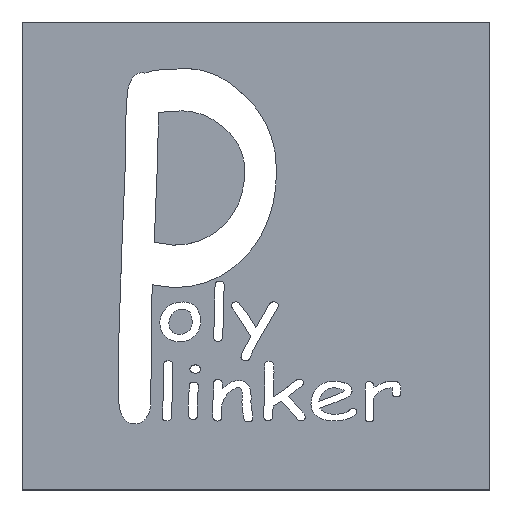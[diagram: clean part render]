
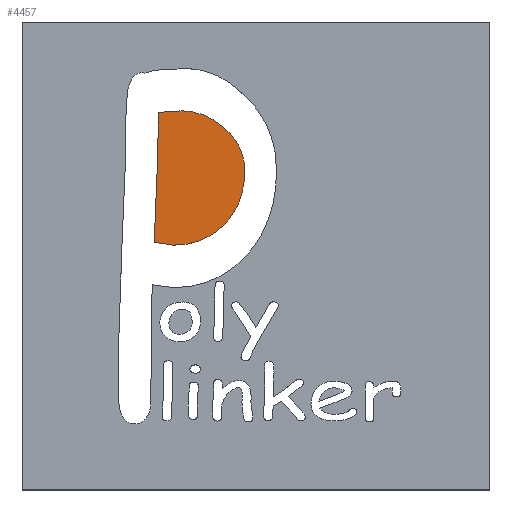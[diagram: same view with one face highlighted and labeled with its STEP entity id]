
A CAD part, top view. The second image highlights one B-rep face of the part: STEP entity #4457.
In plain terms, the highlighted planar face has unit normal (0, 0, 1).
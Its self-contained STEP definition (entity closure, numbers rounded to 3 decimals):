
#68 = EDGE_CURVE ( 'NONE', #655, #737, #5095, .T. ) ;
#99 = FACE_OUTER_BOUND ( 'NONE', #6360, .T. ) ;
#329 = B_SPLINE_CURVE_WITH_KNOTS ( 'NONE', 3,
 ( #1720, #4419, #2565, #1857 ),
 .UNSPECIFIED., .F., .F.,
 ( 4, 4 ),
 ( 0., 1. ),
 .UNSPECIFIED. ) ;
#407 = CARTESIAN_POINT ( 'NONE',  ( -11.199, 9.246, 22.127 ) ) ;
#552 = VECTOR ( 'NONE', #1691, 1000. ) ;
#575 = VECTOR ( 'NONE', #4818, 1000. ) ;
#655 = VERTEX_POINT ( 'NONE', #2930 ) ;
#659 = CARTESIAN_POINT ( 'NONE',  ( -5.569, 11.492, 22.127 ) ) ;
#734 = CARTESIAN_POINT ( 'NONE',  ( -10.305, 12.862, 22.127 ) ) ;
#737 = VERTEX_POINT ( 'NONE', #407 ) ;
#823 = EDGE_CURVE ( 'NONE', #4748, #655, #2637, .T. ) ;
#871 = EDGE_CURVE ( 'NONE', #737, #2828, #1374, .T. ) ;
#1062 = CARTESIAN_POINT ( 'NONE',  ( -7.858, 12.9, 22.127 ) ) ;
#1065 = ORIENTED_EDGE ( 'NONE', *, *, #4635, .T. ) ;
#1147 = EDGE_CURVE ( 'NONE', #3912, #3196, #5154, .T. ) ;
#1374 = LINE ( 'NONE', #3438, #575 ) ;
#1389 = DIRECTION ( 'NONE',  ( 0., 0., -1. ) ) ;
#1469 = DIRECTION ( 'NONE',  ( -1., 0., 0. ) ) ;
#1534 = CARTESIAN_POINT ( 'NONE',  ( -11.511, 1.673, 22.127 ) ) ;
#1585 = EDGE_CURVE ( 'NONE', #2828, #3912, #5687, .T. ) ;
#1691 = DIRECTION ( 'NONE',  ( -0.009, -1., 0. ) ) ;
#1720 = CARTESIAN_POINT ( 'NONE',  ( -5.658, 3.043, 22.127 ) ) ;
#1794 = CARTESIAN_POINT ( 'NONE',  ( -5.658, 3.043, 22.127 ) ) ;
#1857 = CARTESIAN_POINT ( 'NONE',  ( -3.782, 7.819, 22.127 ) ) ;
#1935 = CARTESIAN_POINT ( 'NONE',  ( -5.569, 11.492, 22.127 ) ) ;
#2131 = CARTESIAN_POINT ( 'NONE',  ( 0., 22.127, 22.127 ) ) ;
#2137 = B_SPLINE_CURVE_WITH_KNOTS ( 'NONE', 3,
 ( #8419, #7103, #1062, #7329 ),
 .UNSPECIFIED., .F., .F.,
 ( 4, 4 ),
 ( 0., 1. ),
 .UNSPECIFIED. ) ;
#2221 = CARTESIAN_POINT ( 'NONE',  ( -9.565, 12.9, 22.127 ) ) ;
#2227 = ORIENTED_EDGE ( 'NONE', *, *, #5098, .T. ) ;
#2451 = CARTESIAN_POINT ( 'NONE',  ( -6.8, 1.965, 22.127 ) ) ;
#2565 = CARTESIAN_POINT ( 'NONE',  ( -3.782, 5.815, 22.127 ) ) ;
#2591 = CARTESIAN_POINT ( 'NONE',  ( -8.205, 1.425, 22.127 ) ) ;
#2606 = CARTESIAN_POINT ( 'NONE',  ( -11.511, 1.673, 22.127 ) ) ;
#2637 = B_SPLINE_CURVE_WITH_KNOTS ( 'NONE', 3,
 ( #5141, #7816, #6682, #4480 ),
 .UNSPECIFIED., .F., .F.,
 ( 4, 4 ),
 ( 0., 1. ),
 .UNSPECIFIED. ) ;
#2714 = CARTESIAN_POINT ( 'NONE',  ( -5.658, 3.043, 22.127 ) ) ;
#2750 = PLANE ( 'NONE',  #7639 ) ;
#2828 = VERTEX_POINT ( 'NONE', #2606 ) ;
#2930 = CARTESIAN_POINT ( 'NONE',  ( -11.169, 12.748, 22.127 ) ) ;
#3049 = CARTESIAN_POINT ( 'NONE',  ( -11.169, 12.748, 22.127 ) ) ;
#3060 = DIRECTION ( 'NONE',  ( 0.989, -0.149, 0. ) ) ;
#3166 = ORIENTED_EDGE ( 'NONE', *, *, #68, .T. ) ;
#3196 = VERTEX_POINT ( 'NONE', #2714 ) ;
#3263 = ORIENTED_EDGE ( 'NONE', *, *, #7843, .T. ) ;
#3307 = VERTEX_POINT ( 'NONE', #1935 ) ;
#3438 = CARTESIAN_POINT ( 'NONE',  ( -11.199, 9.246, 22.127 ) ) ;
#3912 = VERTEX_POINT ( 'NONE', #4917 ) ;
#4015 = CARTESIAN_POINT ( 'NONE',  ( -3.782, 9.24, 22.127 ) ) ;
#4145 = B_SPLINE_CURVE_WITH_KNOTS ( 'NONE', 3,
 ( #5347, #4015, #6568, #659 ),
 .UNSPECIFIED., .F., .F.,
 ( 4, 4 ),
 ( 0., 1. ),
 .UNSPECIFIED. ) ;
#4293 = CARTESIAN_POINT ( 'NONE',  ( -3.782, 7.819, 22.127 ) ) ;
#4419 = CARTESIAN_POINT ( 'NONE',  ( -4.407, 4.223, 22.127 ) ) ;
#4449 = ORIENTED_EDGE ( 'NONE', *, *, #871, .T. ) ;
#4457 = ADVANCED_FACE ( 'NONE', ( #99 ), #2750, .F. ) ;
#4480 = CARTESIAN_POINT ( 'NONE',  ( -11.169, 12.748, 22.127 ) ) ;
#4589 = ORIENTED_EDGE ( 'NONE', *, *, #823, .T. ) ;
#4635 = EDGE_CURVE ( 'NONE', #3196, #6566, #329, .T. ) ;
#4691 = ORIENTED_EDGE ( 'NONE', *, *, #8310, .T. ) ;
#4748 = VERTEX_POINT ( 'NONE', #6674 ) ;
#4803 = CARTESIAN_POINT ( 'NONE',  ( -9.957, 12.887, 22.127 ) ) ;
#4818 = DIRECTION ( 'NONE',  ( -0.041, -0.999, 0. ) ) ;
#4917 = CARTESIAN_POINT ( 'NONE',  ( -9.873, 1.425, 22.127 ) ) ;
#5095 = LINE ( 'NONE', #3049, #552 ) ;
#5098 = EDGE_CURVE ( 'NONE', #5437, #4748, #7163, .T. ) ;
#5141 = CARTESIAN_POINT ( 'NONE',  ( -10.305, 12.862, 22.127 ) ) ;
#5154 = B_SPLINE_CURVE_WITH_KNOTS ( 'NONE', 3,
 ( #7227, #2591, #2451, #1794 ),
 .UNSPECIFIED., .F., .F.,
 ( 4, 4 ),
 ( 0., 1. ),
 .UNSPECIFIED. ) ;
#5347 = CARTESIAN_POINT ( 'NONE',  ( -3.782, 7.819, 22.127 ) ) ;
#5437 = VERTEX_POINT ( 'NONE', #7738 ) ;
#5687 = LINE ( 'NONE', #1534, #7470 ) ;
#6360 = EDGE_LOOP ( 'NONE', ( #3263, #2227, #4589, #3166, #4449, #8290, #8255, #1065, #4691 ) ) ;
#6566 = VERTEX_POINT ( 'NONE', #4293 ) ;
#6568 = CARTESIAN_POINT ( 'NONE',  ( -4.377, 10.464, 22.127 ) ) ;
#6674 = CARTESIAN_POINT ( 'NONE',  ( -10.305, 12.862, 22.127 ) ) ;
#6682 = CARTESIAN_POINT ( 'NONE',  ( -10.931, 12.798, 22.127 ) ) ;
#7103 = CARTESIAN_POINT ( 'NONE',  ( -6.671, 12.43, 22.127 ) ) ;
#7163 = B_SPLINE_CURVE_WITH_KNOTS ( 'NONE', 3,
 ( #7599, #2221, #4803, #734 ),
 .UNSPECIFIED., .F., .F.,
 ( 4, 4 ),
 ( 0., 1. ),
 .UNSPECIFIED. ) ;
#7227 = CARTESIAN_POINT ( 'NONE',  ( -9.873, 1.425, 22.127 ) ) ;
#7329 = CARTESIAN_POINT ( 'NONE',  ( -9.128, 12.9, 22.127 ) ) ;
#7470 = VECTOR ( 'NONE', #3060, 1000. ) ;
#7599 = CARTESIAN_POINT ( 'NONE',  ( -9.128, 12.9, 22.127 ) ) ;
#7639 = AXIS2_PLACEMENT_3D ( 'NONE', #2131, #1389, #1469 ) ;
#7738 = CARTESIAN_POINT ( 'NONE',  ( -9.128, 12.9, 22.127 ) ) ;
#7816 = CARTESIAN_POINT ( 'NONE',  ( -10.643, 12.836, 22.127 ) ) ;
#7843 = EDGE_CURVE ( 'NONE', #3307, #5437, #2137, .T. ) ;
#8255 = ORIENTED_EDGE ( 'NONE', *, *, #1147, .T. ) ;
#8290 = ORIENTED_EDGE ( 'NONE', *, *, #1585, .T. ) ;
#8310 = EDGE_CURVE ( 'NONE', #6566, #3307, #4145, .T. ) ;
#8419 = CARTESIAN_POINT ( 'NONE',  ( -5.569, 11.492, 22.127 ) ) ;
